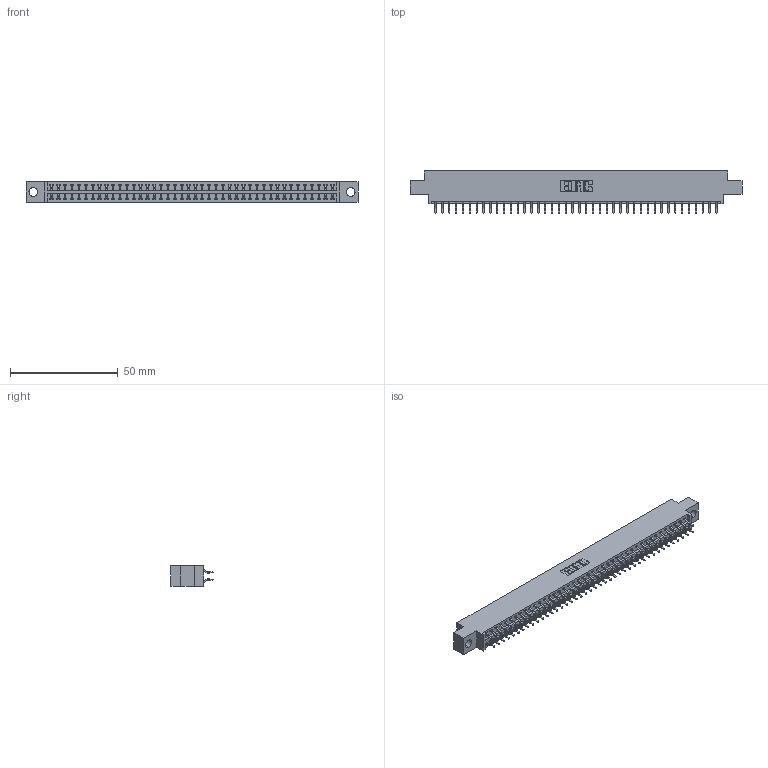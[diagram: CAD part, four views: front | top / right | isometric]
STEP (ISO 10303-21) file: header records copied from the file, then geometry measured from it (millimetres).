
FILE_DESCRIPTION (( 'STEP AP203' ), '1' );
FILE_NAME ('346-084-556-804.STEP', '2022-05-25T20:43:15', ( '' ), ( '' ), 'SwSTEP 2.0', 'SolidWorks 2020', '' );
FILE_SCHEMA (( 'CONFIG_CONTROL_DESIGN' ));
Length unit declared in the file: inch
Products named in the file (3): 345-292-001_556 Tail; 346 Part_0.170 Offset - 0.156 Dia-TH; 346-084-556-804
Assembly tree (85 placements, depth 2):
  346-084-556-804
    346 Part_0.170 Offset - 0.156 Dia-TH
    345-292-001_556 Tail  x84
Bounding box: 153.92 x 19.57 x 9.4 mm (x, y, z)
Volume: 14745.6 mm3; surface area: 20218.3 mm2
Topology: 85 solids, 85 shells, 5012 faces, 14909 edges, 9826 vertices
Faces by surface type: plane 3370, cylinder 1642
Entity records: 28181 total; most frequent: CARTESIAN_POINT 4666, ORIENTED_EDGE 4586, DIRECTION 4149, EDGE_CURVE 2293, VECTOR 1985, LINE 1985, VERTEX_POINT 1526, AXIS2_PLACEMENT_3D 1082
